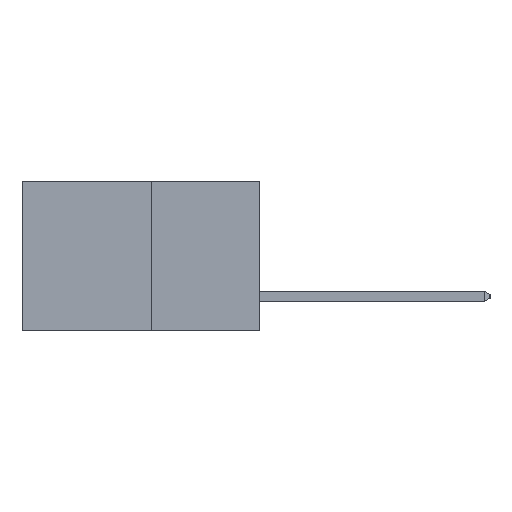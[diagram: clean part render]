
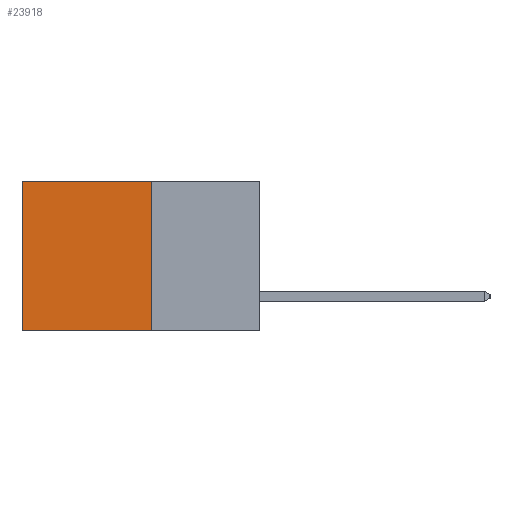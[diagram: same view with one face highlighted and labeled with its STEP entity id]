
A CAD part, left-side view. The second image highlights one B-rep face of the part: STEP entity #23918.
In plain terms, the highlighted planar face has unit normal (-1, 0, 0).
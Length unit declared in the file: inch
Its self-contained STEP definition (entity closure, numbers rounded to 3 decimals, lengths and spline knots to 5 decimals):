
#719 = EDGE_CURVE ( 'NONE', #18318, #1556, #8390, .T. ) ;
#762 = LINE ( 'NONE', #19641, #9885 ) ;
#947 = CARTESIAN_POINT ( 'NONE',  ( 0.277, 0.59, -0.37 ) ) ;
#1556 = VERTEX_POINT ( 'NONE', #947 ) ;
#2356 = CARTESIAN_POINT ( 'NONE',  ( 0.277, 0.27, -0.37 ) ) ;
#2586 = FACE_OUTER_BOUND ( 'NONE', #4465, .T. ) ;
#2629 = ORIENTED_EDGE ( 'NONE', *, *, #24173, .F. ) ;
#2948 = DIRECTION ( 'NONE',  ( 0., 1., 0. ) ) ;
#2981 = VERTEX_POINT ( 'NONE', #13064 ) ;
#3250 = AXIS2_PLACEMENT_3D ( 'NONE', #4786, #18264, #6747 ) ;
#4465 = EDGE_LOOP ( 'NONE', ( #21673, #20146, #2629, #5737 ) ) ;
#4786 = CARTESIAN_POINT ( 'NONE',  ( 0.277, 0.27, -0.37 ) ) ;
#5737 = ORIENTED_EDGE ( 'NONE', *, *, #8074, .T. ) ;
#5776 = VERTEX_POINT ( 'NONE', #15204 ) ;
#6237 = LINE ( 'NONE', #9433, #15880 ) ;
#6747 = DIRECTION ( 'NONE',  ( 0., 0., -1. ) ) ;
#8074 = EDGE_CURVE ( 'NONE', #5776, #2981, #9642, .T. ) ;
#8390 = LINE ( 'NONE', #8703, #13537 ) ;
#8703 = CARTESIAN_POINT ( 'NONE',  ( 0.277, 0.27, -0.37 ) ) ;
#9433 = CARTESIAN_POINT ( 'NONE',  ( 0.277, 0.27, -0.37 ) ) ;
#9642 = LINE ( 'NONE', #10700, #24191 ) ;
#9885 = VECTOR ( 'NONE', #21524, 39.37008 ) ;
#10700 = CARTESIAN_POINT ( 'NONE',  ( 0.277, 0.27, 0. ) ) ;
#11377 = DIRECTION ( 'NONE',  ( 0., 0., -1. ) ) ;
#12629 = DIRECTION ( 'NONE',  ( 0., 1., 0. ) ) ;
#13064 = CARTESIAN_POINT ( 'NONE',  ( 0.277, 0.59, 0. ) ) ;
#13537 = VECTOR ( 'NONE', #2948, 39.37008 ) ;
#15204 = CARTESIAN_POINT ( 'NONE',  ( 0.277, 0.27, 0. ) ) ;
#15880 = VECTOR ( 'NONE', #11377, 39.37008 ) ;
#16331 = PLANE ( 'NONE',  #3250 ) ;
#17685 = EDGE_CURVE ( 'NONE', #2981, #1556, #762, .T. ) ;
#18264 = DIRECTION ( 'NONE',  ( 1., 0., 0. ) ) ;
#18318 = VERTEX_POINT ( 'NONE', #2356 ) ;
#19641 = CARTESIAN_POINT ( 'NONE',  ( 0.277, 0.59, -0.37 ) ) ;
#20146 = ORIENTED_EDGE ( 'NONE', *, *, #719, .F. ) ;
#21524 = DIRECTION ( 'NONE',  ( 0., 0., -1. ) ) ;
#21673 = ORIENTED_EDGE ( 'NONE', *, *, #17685, .T. ) ;
#23918 = ADVANCED_FACE ( 'NONE', ( #2586 ), #16331, .F. ) ;
#24173 = EDGE_CURVE ( 'NONE', #5776, #18318, #6237, .T. ) ;
#24191 = VECTOR ( 'NONE', #12629, 39.37008 ) ;
